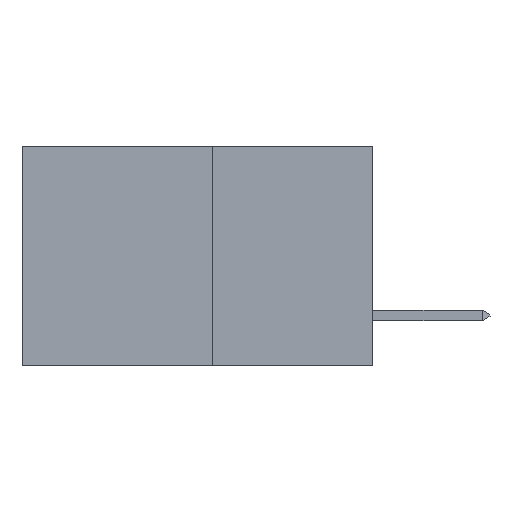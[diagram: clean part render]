
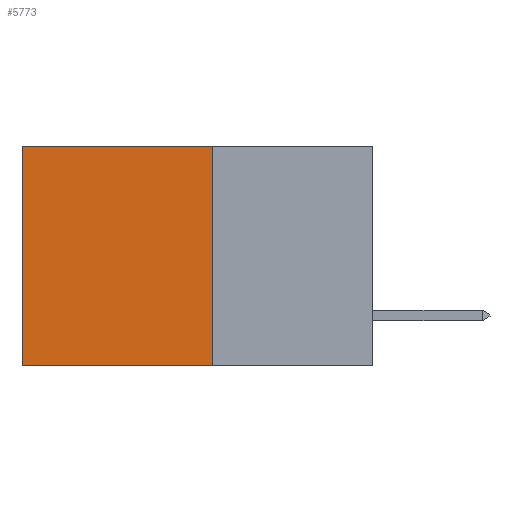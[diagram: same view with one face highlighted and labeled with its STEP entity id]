
A CAD part, left-side view. The second image highlights one B-rep face of the part: STEP entity #5773.
In plain terms, the highlighted planar face has unit normal (-1, 0, 0).
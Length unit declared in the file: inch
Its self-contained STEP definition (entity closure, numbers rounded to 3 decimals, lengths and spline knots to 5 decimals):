
#34 = CARTESIAN_POINT ( 'NONE',  ( 0.277, 0.27, 0. ) ) ;
#35 = ORIENTED_EDGE ( 'NONE', *, *, #1064, .T. ) ;
#284 = CARTESIAN_POINT ( 'NONE',  ( 0.277, 0.27, -0.37 ) ) ;
#492 = VECTOR ( 'NONE', #8709, 39.37008 ) ;
#505 = CARTESIAN_POINT ( 'NONE',  ( 0.277, 0.27, -0.37 ) ) ;
#572 = VERTEX_POINT ( 'NONE', #5241 ) ;
#694 = LINE ( 'NONE', #7966, #492 ) ;
#700 = CARTESIAN_POINT ( 'NONE',  ( 0.277, 0.27, -0.37 ) ) ;
#815 = DIRECTION ( 'NONE',  ( 0., 0., -1. ) ) ;
#1064 = EDGE_CURVE ( 'NONE', #4699, #7855, #1461, .T. ) ;
#1092 = DIRECTION ( 'NONE',  ( 0., 0., -1. ) ) ;
#1094 = LINE ( 'NONE', #1971, #6392 ) ;
#1168 = DIRECTION ( 'NONE',  ( 1., 0., 0. ) ) ;
#1178 = EDGE_LOOP ( 'NONE', ( #3144, #4202, #3493, #35 ) ) ;
#1235 = PLANE ( 'NONE',  #2270 ) ;
#1461 = LINE ( 'NONE', #34, #8540 ) ;
#1971 = CARTESIAN_POINT ( 'NONE',  ( 0.277, 0.59, -0.37 ) ) ;
#2154 = LINE ( 'NONE', #284, #5435 ) ;
#2175 = CARTESIAN_POINT ( 'NONE',  ( 0.277, 0.59, 0. ) ) ;
#2270 = AXIS2_PLACEMENT_3D ( 'NONE', #505, #1168, #1092 ) ;
#3144 = ORIENTED_EDGE ( 'NONE', *, *, #4582, .T. ) ;
#3493 = ORIENTED_EDGE ( 'NONE', *, *, #6817, .F. ) ;
#4202 = ORIENTED_EDGE ( 'NONE', *, *, #6608, .F. ) ;
#4582 = EDGE_CURVE ( 'NONE', #7855, #572, #1094, .T. ) ;
#4699 = VERTEX_POINT ( 'NONE', #7838 ) ;
#5146 = DIRECTION ( 'NONE',  ( 0., 1., 0. ) ) ;
#5241 = CARTESIAN_POINT ( 'NONE',  ( 0.277, 0.59, -0.37 ) ) ;
#5435 = VECTOR ( 'NONE', #8348, 39.37008 ) ;
#5773 = ADVANCED_FACE ( 'NONE', ( #6517 ), #1235, .F. ) ;
#6392 = VECTOR ( 'NONE', #815, 39.37008 ) ;
#6517 = FACE_OUTER_BOUND ( 'NONE', #1178, .T. ) ;
#6563 = VERTEX_POINT ( 'NONE', #700 ) ;
#6608 = EDGE_CURVE ( 'NONE', #6563, #572, #694, .T. ) ;
#6817 = EDGE_CURVE ( 'NONE', #4699, #6563, #2154, .T. ) ;
#7838 = CARTESIAN_POINT ( 'NONE',  ( 0.277, 0.27, 0. ) ) ;
#7855 = VERTEX_POINT ( 'NONE', #2175 ) ;
#7966 = CARTESIAN_POINT ( 'NONE',  ( 0.277, 0.27, -0.37 ) ) ;
#8348 = DIRECTION ( 'NONE',  ( 0., 0., -1. ) ) ;
#8540 = VECTOR ( 'NONE', #5146, 39.37008 ) ;
#8709 = DIRECTION ( 'NONE',  ( 0., 1., 0. ) ) ;
